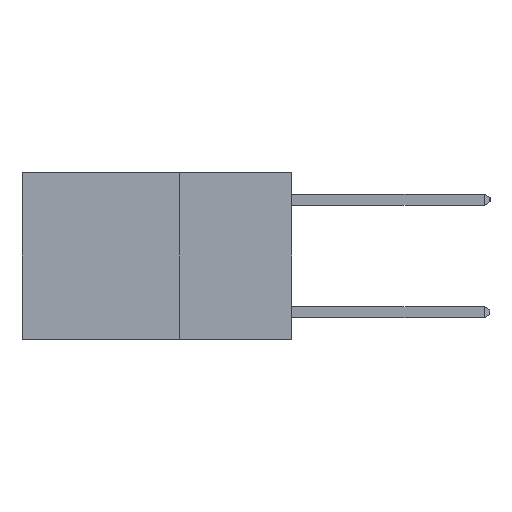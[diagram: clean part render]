
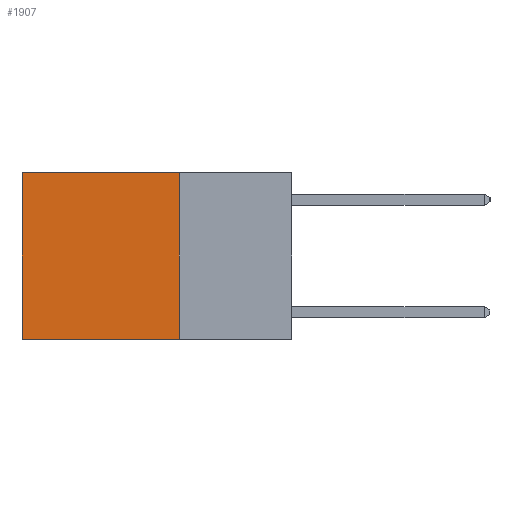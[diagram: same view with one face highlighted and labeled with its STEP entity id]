
A CAD part, left-side view. The second image highlights one B-rep face of the part: STEP entity #1907.
In plain terms, the highlighted planar face has unit normal (-1, 0, 0).
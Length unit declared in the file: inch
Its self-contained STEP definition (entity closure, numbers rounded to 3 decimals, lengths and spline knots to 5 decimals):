
#24 = CARTESIAN_POINT ( 'NONE',  ( 0.2625, 0.25, 0. ) ) ;
#691 = VECTOR ( 'NONE', #4851, 39.37008 ) ;
#926 = DIRECTION ( 'NONE',  ( 0., 0., -1. ) ) ;
#1084 = EDGE_CURVE ( 'NONE', #4445, #11566, #2555, .T. ) ;
#1658 = LINE ( 'NONE', #5645, #4242 ) ;
#1801 = LINE ( 'NONE', #8960, #9091 ) ;
#1907 = ADVANCED_FACE ( 'NONE', ( #1949 ), #9609, .F. ) ;
#1949 = FACE_OUTER_BOUND ( 'NONE', #6225, .T. ) ;
#2555 = LINE ( 'NONE', #6718, #4833 ) ;
#2884 = ORIENTED_EDGE ( 'NONE', *, *, #7162, .T. ) ;
#3278 = LINE ( 'NONE', #9508, #691 ) ;
#4029 = VERTEX_POINT ( 'NONE', #10173 ) ;
#4094 = ORIENTED_EDGE ( 'NONE', *, *, #9470, .F. ) ;
#4242 = VECTOR ( 'NONE', #12130, 39.37008 ) ;
#4445 = VERTEX_POINT ( 'NONE', #11599 ) ;
#4833 = VECTOR ( 'NONE', #926, 39.37008 ) ;
#4851 = DIRECTION ( 'NONE',  ( 0., 1., 0. ) ) ;
#4954 = DIRECTION ( 'NONE',  ( 0., 0., -1. ) ) ;
#5645 = CARTESIAN_POINT ( 'NONE',  ( 0.2625, 0.6, 0. ) ) ;
#6075 = CARTESIAN_POINT ( 'NONE',  ( 0.2625, 0.25, -0.37 ) ) ;
#6225 = EDGE_LOOP ( 'NONE', ( #2884, #4094, #7857, #9423 ) ) ;
#6447 = VERTEX_POINT ( 'NONE', #8354 ) ;
#6718 = CARTESIAN_POINT ( 'NONE',  ( 0.2625, 0.25, 0. ) ) ;
#7162 = EDGE_CURVE ( 'NONE', #6447, #4029, #1658, .T. ) ;
#7857 = ORIENTED_EDGE ( 'NONE', *, *, #1084, .F. ) ;
#7955 = EDGE_CURVE ( 'NONE', #4445, #6447, #1801, .T. ) ;
#8354 = CARTESIAN_POINT ( 'NONE',  ( 0.2625, 0.6, 0. ) ) ;
#8960 = CARTESIAN_POINT ( 'NONE',  ( 0.2625, 0.25, 0. ) ) ;
#9091 = VECTOR ( 'NONE', #9887, 39.37008 ) ;
#9423 = ORIENTED_EDGE ( 'NONE', *, *, #7955, .T. ) ;
#9470 = EDGE_CURVE ( 'NONE', #11566, #4029, #3278, .T. ) ;
#9508 = CARTESIAN_POINT ( 'NONE',  ( 0.2625, 0.25, -0.37 ) ) ;
#9609 = PLANE ( 'NONE',  #10307 ) ;
#9887 = DIRECTION ( 'NONE',  ( 0., 1., 0. ) ) ;
#10173 = CARTESIAN_POINT ( 'NONE',  ( 0.2625, 0.6, -0.37 ) ) ;
#10307 = AXIS2_PLACEMENT_3D ( 'NONE', #24, #10551, #4954 ) ;
#10551 = DIRECTION ( 'NONE',  ( 1., 0., 0. ) ) ;
#11566 = VERTEX_POINT ( 'NONE', #6075 ) ;
#11599 = CARTESIAN_POINT ( 'NONE',  ( 0.2625, 0.25, 0. ) ) ;
#12130 = DIRECTION ( 'NONE',  ( 0., 0., -1. ) ) ;
